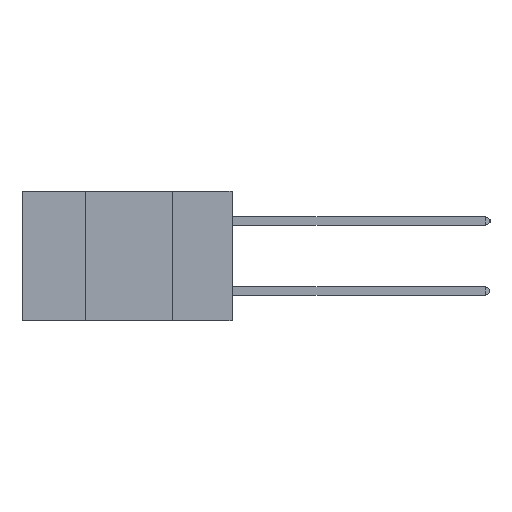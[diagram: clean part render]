
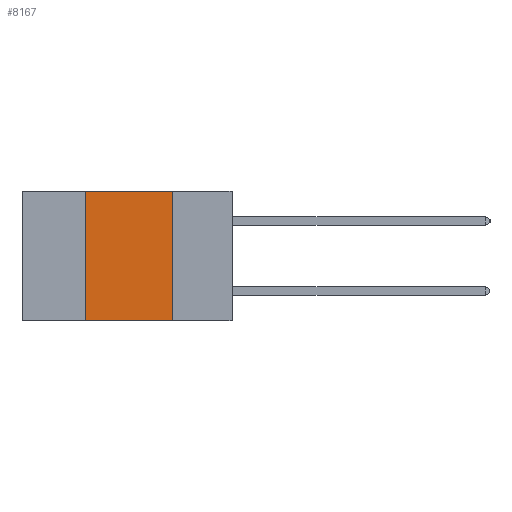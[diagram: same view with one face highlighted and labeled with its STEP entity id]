
A CAD part, left-side view. The second image highlights one B-rep face of the part: STEP entity #8167.
In plain terms, the highlighted planar face has unit normal (-1, 0, 0).
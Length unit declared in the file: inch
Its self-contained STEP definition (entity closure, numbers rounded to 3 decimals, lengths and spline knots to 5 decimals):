
#48 = CARTESIAN_POINT ( 'NONE',  ( 0., 0.17, 0. ) ) ;
#435 = CARTESIAN_POINT ( 'NONE',  ( 0., 0.42, 0. ) ) ;
#544 = EDGE_CURVE ( 'NONE', #3447, #3064, #10886, .T. ) ;
#834 = CARTESIAN_POINT ( 'NONE',  ( 0., 0.42, -0.37 ) ) ;
#1182 = EDGE_CURVE ( 'NONE', #11621, #3064, #6525, .T. ) ;
#1356 = EDGE_LOOP ( 'NONE', ( #3716, #3730, #3747, #3836 ) ) ;
#2199 = CARTESIAN_POINT ( 'NONE',  ( 0., 0.6, 0. ) ) ;
#2709 = VECTOR ( 'NONE', #10926, 39.37008 ) ;
#2742 = VERTEX_POINT ( 'NONE', #435 ) ;
#2862 = VECTOR ( 'NONE', #4074, 39.37008 ) ;
#3064 = VERTEX_POINT ( 'NONE', #11892 ) ;
#3183 = DIRECTION ( 'NONE',  ( 0., 0., -1. ) ) ;
#3447 = VERTEX_POINT ( 'NONE', #834 ) ;
#3576 = EDGE_CURVE ( 'NONE', #3447, #2742, #5580, .T. ) ;
#3716 = ORIENTED_EDGE ( 'NONE', *, *, #1182, .F. ) ;
#3730 = ORIENTED_EDGE ( 'NONE', *, *, #12632, .F. ) ;
#3747 = ORIENTED_EDGE ( 'NONE', *, *, #3576, .F. ) ;
#3836 = ORIENTED_EDGE ( 'NONE', *, *, #544, .T. ) ;
#3950 = DIRECTION ( 'NONE',  ( 0., 0., -1. ) ) ;
#4036 = DIRECTION ( 'NONE',  ( 0., -1., 0. ) ) ;
#4045 = AXIS2_PLACEMENT_3D ( 'NONE', #8641, #9680, #3183 ) ;
#4074 = DIRECTION ( 'NONE',  ( 0., 0., 1. ) ) ;
#4323 = PLANE ( 'NONE',  #4045 ) ;
#5580 = LINE ( 'NONE', #10460, #2862 ) ;
#6027 = VECTOR ( 'NONE', #4036, 39.37008 ) ;
#6525 = LINE ( 'NONE', #48, #12351 ) ;
#8167 = ADVANCED_FACE ( 'NONE', ( #10796 ), #4323, .F. ) ;
#8641 = CARTESIAN_POINT ( 'NONE',  ( 0., 0.6, 0. ) ) ;
#9680 = DIRECTION ( 'NONE',  ( 1., 0., 0. ) ) ;
#10460 = CARTESIAN_POINT ( 'NONE',  ( 0., 0.42, 0. ) ) ;
#10796 = FACE_OUTER_BOUND ( 'NONE', #1356, .T. ) ;
#10886 = LINE ( 'NONE', #11311, #6027 ) ;
#10926 = DIRECTION ( 'NONE',  ( 0., -1., 0. ) ) ;
#11135 = CARTESIAN_POINT ( 'NONE',  ( 0., 0.17, 0. ) ) ;
#11311 = CARTESIAN_POINT ( 'NONE',  ( 0., 0.6, -0.37 ) ) ;
#11348 = LINE ( 'NONE', #2199, #2709 ) ;
#11621 = VERTEX_POINT ( 'NONE', #11135 ) ;
#11892 = CARTESIAN_POINT ( 'NONE',  ( 0., 0.17, -0.37 ) ) ;
#12351 = VECTOR ( 'NONE', #3950, 39.37008 ) ;
#12632 = EDGE_CURVE ( 'NONE', #2742, #11621, #11348, .T. ) ;
